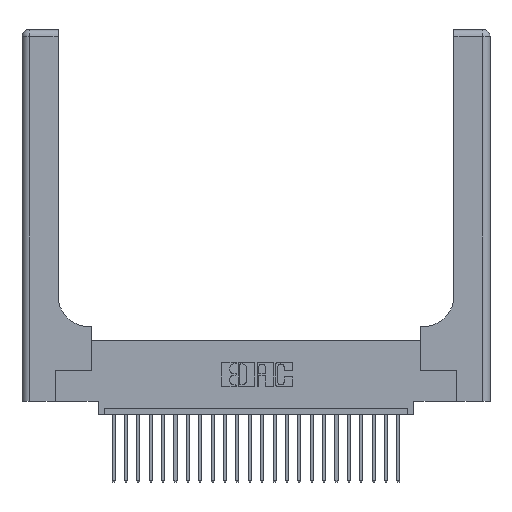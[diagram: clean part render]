
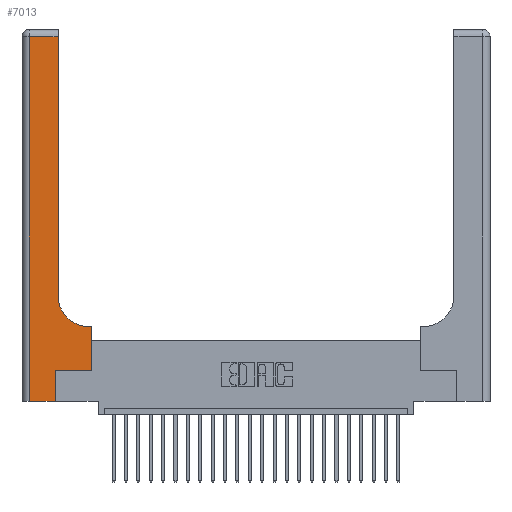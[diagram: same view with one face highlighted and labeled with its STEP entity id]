
A CAD part, top view. The second image highlights one B-rep face of the part: STEP entity #7013.
In plain terms, the highlighted planar face has unit normal (0, 0, 1).
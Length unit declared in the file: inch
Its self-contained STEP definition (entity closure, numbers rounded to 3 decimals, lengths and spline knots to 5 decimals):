
#371 = DIRECTION ( 'NONE',  ( 0., 1., 0. ) ) ;
#1737 = VECTOR ( 'NONE', #371, 39.37008 ) ;
#1744 = CARTESIAN_POINT ( 'NONE',  ( 0.269, 0., 0.37 ) ) ;
#1882 = DIRECTION ( 'NONE',  ( 0., 0., -1. ) ) ;
#2105 = VERTEX_POINT ( 'NONE', #25067 ) ;
#2395 = LINE ( 'NONE', #15226, #7745 ) ;
#2837 = ORIENTED_EDGE ( 'NONE', *, *, #19894, .T. ) ;
#3756 = LINE ( 'NONE', #9563, #24309 ) ;
#3767 = LINE ( 'NONE', #8493, #23726 ) ;
#3961 = VERTEX_POINT ( 'NONE', #13682 ) ;
#4229 = CARTESIAN_POINT ( 'NONE',  ( 0.2915, 3., 0.37 ) ) ;
#4512 = DIRECTION ( 'NONE',  ( 1., 0., 0. ) ) ;
#4650 = DIRECTION ( 'NONE',  ( 0., 1., 0. ) ) ;
#5678 = ORIENTED_EDGE ( 'NONE', *, *, #21279, .T. ) ;
#5995 = DIRECTION ( 'NONE',  ( 1., 0., 0. ) ) ;
#6078 = DIRECTION ( 'NONE',  ( -1., 0., 0. ) ) ;
#6429 = VECTOR ( 'NONE', #4512, 39.37008 ) ;
#7013 = ADVANCED_FACE ( 'NONE', ( #24193 ), #10035, .F. ) ;
#7190 = EDGE_CURVE ( 'NONE', #2105, #23725, #9888, .T. ) ;
#7745 = VECTOR ( 'NONE', #23078, 39.37008 ) ;
#7856 = CARTESIAN_POINT ( 'NONE',  ( 0., 3., 0.37 ) ) ;
#7877 = CARTESIAN_POINT ( 'NONE',  ( 0.269, 0.25, 0.37 ) ) ;
#8003 = DIRECTION ( 'NONE',  ( 0., 1., 0. ) ) ;
#8126 = ORIENTED_EDGE ( 'NONE', *, *, #12886, .T. ) ;
#8226 = EDGE_CURVE ( 'NONE', #18021, #2105, #25065, .T. ) ;
#8493 = CARTESIAN_POINT ( 'NONE',  ( 0., 2.94, 0.37 ) ) ;
#9150 = CARTESIAN_POINT ( 'NONE',  ( 0.06, 2.94, 0.37 ) ) ;
#9563 = CARTESIAN_POINT ( 'NONE',  ( 0., 0., 0.37 ) ) ;
#9888 = LINE ( 'NONE', #4229, #1737 ) ;
#10035 = PLANE ( 'NONE',  #18607 ) ;
#10130 = VERTEX_POINT ( 'NONE', #1744 ) ;
#10131 = CARTESIAN_POINT ( 'NONE',  ( 0.5415, 0.85, 0.37 ) ) ;
#10794 = VERTEX_POINT ( 'NONE', #21484 ) ;
#11499 = CARTESIAN_POINT ( 'NONE',  ( 0.2915, 0.6, 0.37 ) ) ;
#11547 = VERTEX_POINT ( 'NONE', #21642 ) ;
#11684 = VECTOR ( 'NONE', #8003, 39.37008 ) ;
#12032 = EDGE_CURVE ( 'NONE', #11547, #18021, #20882, .T. ) ;
#12383 = LINE ( 'NONE', #13269, #6429 ) ;
#12886 = EDGE_CURVE ( 'NONE', #22549, #10794, #2395, .T. ) ;
#13243 = ORIENTED_EDGE ( 'NONE', *, *, #24914, .T. ) ;
#13269 = CARTESIAN_POINT ( 'NONE',  ( 0.269, 0.25, 0.37 ) ) ;
#13311 = CARTESIAN_POINT ( 'NONE',  ( 0.5415, 0.6, 0.37 ) ) ;
#13682 = CARTESIAN_POINT ( 'NONE',  ( 0.5585, 0.25, 0.37 ) ) ;
#14895 = LINE ( 'NONE', #16599, #24806 ) ;
#14998 = EDGE_CURVE ( 'NONE', #23725, #22549, #3767, .T. ) ;
#15226 = CARTESIAN_POINT ( 'NONE',  ( 0.06, 3., 0.37 ) ) ;
#15913 = ORIENTED_EDGE ( 'NONE', *, *, #17723, .T. ) ;
#16599 = CARTESIAN_POINT ( 'NONE',  ( 0.5585, 0.25, 0.37 ) ) ;
#16810 = ORIENTED_EDGE ( 'NONE', *, *, #7190, .T. ) ;
#16876 = DIRECTION ( 'NONE',  ( -1., 0., 0. ) ) ;
#17723 = EDGE_CURVE ( 'NONE', #17768, #3961, #12383, .T. ) ;
#17768 = VERTEX_POINT ( 'NONE', #7877 ) ;
#18021 = VERTEX_POINT ( 'NONE', #13311 ) ;
#18607 = AXIS2_PLACEMENT_3D ( 'NONE', #7856, #1882, #6078 ) ;
#18738 = ORIENTED_EDGE ( 'NONE', *, *, #12032, .T. ) ;
#19894 = EDGE_CURVE ( 'NONE', #10130, #17768, #24391, .T. ) ;
#19920 = CARTESIAN_POINT ( 'NONE',  ( 0.269, 0., 0.37 ) ) ;
#20882 = LINE ( 'NONE', #11499, #23669 ) ;
#21279 = EDGE_CURVE ( 'NONE', #3961, #11547, #14895, .T. ) ;
#21484 = CARTESIAN_POINT ( 'NONE',  ( 0.06, 0., 0.37 ) ) ;
#21642 = CARTESIAN_POINT ( 'NONE',  ( 0.5585, 0.6, 0.37 ) ) ;
#21681 = EDGE_LOOP ( 'NONE', ( #16810, #22163, #8126, #13243, #2837, #15913, #5678, #18738, #25378 ) ) ;
#21900 = DIRECTION ( 'NONE',  ( 0., 0., -1. ) ) ;
#22163 = ORIENTED_EDGE ( 'NONE', *, *, #14998, .T. ) ;
#22549 = VERTEX_POINT ( 'NONE', #9150 ) ;
#23078 = DIRECTION ( 'NONE',  ( 0., -1., 0. ) ) ;
#23455 = AXIS2_PLACEMENT_3D ( 'NONE', #10131, #21900, #5995 ) ;
#23583 = DIRECTION ( 'NONE',  ( -1., 0., 0. ) ) ;
#23669 = VECTOR ( 'NONE', #23583, 39.37008 ) ;
#23725 = VERTEX_POINT ( 'NONE', #25500 ) ;
#23726 = VECTOR ( 'NONE', #16876, 39.37008 ) ;
#24193 = FACE_OUTER_BOUND ( 'NONE', #21681, .T. ) ;
#24309 = VECTOR ( 'NONE', #25524, 39.37008 ) ;
#24391 = LINE ( 'NONE', #19920, #11684 ) ;
#24806 = VECTOR ( 'NONE', #4650, 39.37008 ) ;
#24914 = EDGE_CURVE ( 'NONE', #10794, #10130, #3756, .T. ) ;
#25065 = CIRCLE ( 'NONE', #23455, 0.25 ) ;
#25067 = CARTESIAN_POINT ( 'NONE',  ( 0.2915, 0.85, 0.37 ) ) ;
#25378 = ORIENTED_EDGE ( 'NONE', *, *, #8226, .T. ) ;
#25500 = CARTESIAN_POINT ( 'NONE',  ( 0.2915, 2.94, 0.37 ) ) ;
#25524 = DIRECTION ( 'NONE',  ( 1., 0., 0. ) ) ;
